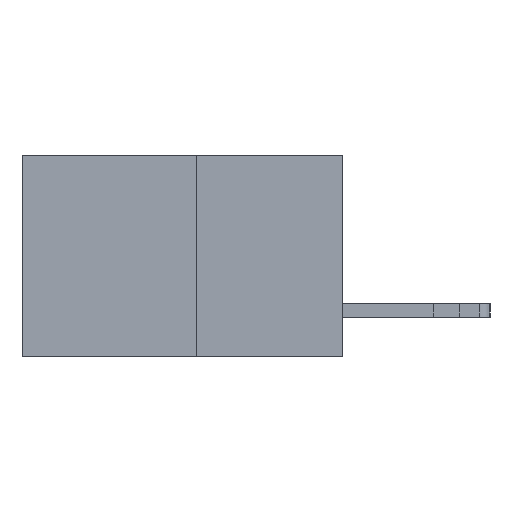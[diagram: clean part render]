
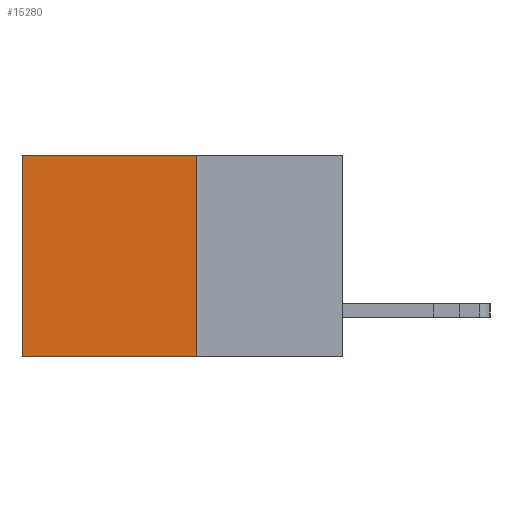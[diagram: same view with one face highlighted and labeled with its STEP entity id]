
A CAD part, left-side view. The second image highlights one B-rep face of the part: STEP entity #15280.
In plain terms, the highlighted planar face has unit normal (-1, 0, 0).
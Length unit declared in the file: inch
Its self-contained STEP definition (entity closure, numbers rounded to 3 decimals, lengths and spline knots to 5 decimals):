
#155 = ORIENTED_EDGE ( 'NONE', *, *, #10382, .F. ) ;
#2244 = AXIS2_PLACEMENT_3D ( 'NONE', #19750, #15136, #5652 ) ;
#2277 = LINE ( 'NONE', #12299, #18102 ) ;
#4770 = LINE ( 'NONE', #7170, #16900 ) ;
#4998 = CARTESIAN_POINT ( 'NONE',  ( 0.277, 0.27, -0.37 ) ) ;
#5431 = CARTESIAN_POINT ( 'NONE',  ( 0.277, 0.27, -0.37 ) ) ;
#5539 = FACE_OUTER_BOUND ( 'NONE', #18465, .T. ) ;
#5652 = DIRECTION ( 'NONE',  ( 0., 0., -1. ) ) ;
#5887 = LINE ( 'NONE', #5431, #13823 ) ;
#7170 = CARTESIAN_POINT ( 'NONE',  ( 0.277, 0.27, -0.37 ) ) ;
#7493 = CARTESIAN_POINT ( 'NONE',  ( 0.277, 0.59, -0.37 ) ) ;
#7573 = DIRECTION ( 'NONE',  ( 0., 1., 0. ) ) ;
#7877 = VECTOR ( 'NONE', #9080, 39.37008 ) ;
#8624 = VERTEX_POINT ( 'NONE', #9382 ) ;
#8745 = DIRECTION ( 'NONE',  ( 0., 1., 0. ) ) ;
#8904 = CARTESIAN_POINT ( 'NONE',  ( 0.277, 0.27, 0. ) ) ;
#9080 = DIRECTION ( 'NONE',  ( 0., 0., -1. ) ) ;
#9382 = CARTESIAN_POINT ( 'NONE',  ( 0.277, 0.59, -0.37 ) ) ;
#10382 = EDGE_CURVE ( 'NONE', #20102, #8624, #4770, .T. ) ;
#10546 = EDGE_CURVE ( 'NONE', #12613, #16655, #2277, .T. ) ;
#12299 = CARTESIAN_POINT ( 'NONE',  ( 0.277, 0.27, 0. ) ) ;
#12613 = VERTEX_POINT ( 'NONE', #8904 ) ;
#12654 = ORIENTED_EDGE ( 'NONE', *, *, #17874, .T. ) ;
#13156 = EDGE_CURVE ( 'NONE', #12613, #20102, #5887, .T. ) ;
#13356 = ORIENTED_EDGE ( 'NONE', *, *, #13156, .F. ) ;
#13547 = PLANE ( 'NONE',  #2244 ) ;
#13823 = VECTOR ( 'NONE', #19622, 39.37008 ) ;
#14914 = ORIENTED_EDGE ( 'NONE', *, *, #10546, .T. ) ;
#15136 = DIRECTION ( 'NONE',  ( 1., 0., 0. ) ) ;
#15280 = ADVANCED_FACE ( 'NONE', ( #5539 ), #13547, .F. ) ;
#16294 = LINE ( 'NONE', #7493, #7877 ) ;
#16655 = VERTEX_POINT ( 'NONE', #19895 ) ;
#16900 = VECTOR ( 'NONE', #8745, 39.37008 ) ;
#17874 = EDGE_CURVE ( 'NONE', #16655, #8624, #16294, .T. ) ;
#18102 = VECTOR ( 'NONE', #7573, 39.37008 ) ;
#18465 = EDGE_LOOP ( 'NONE', ( #12654, #155, #13356, #14914 ) ) ;
#19622 = DIRECTION ( 'NONE',  ( 0., 0., -1. ) ) ;
#19750 = CARTESIAN_POINT ( 'NONE',  ( 0.277, 0.27, -0.37 ) ) ;
#19895 = CARTESIAN_POINT ( 'NONE',  ( 0.277, 0.59, 0. ) ) ;
#20102 = VERTEX_POINT ( 'NONE', #4998 ) ;
